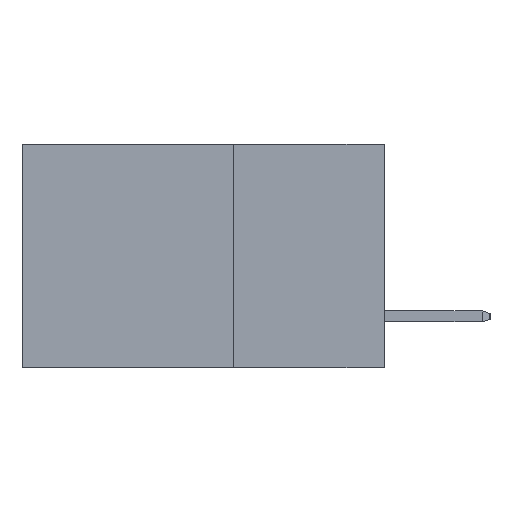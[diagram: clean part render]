
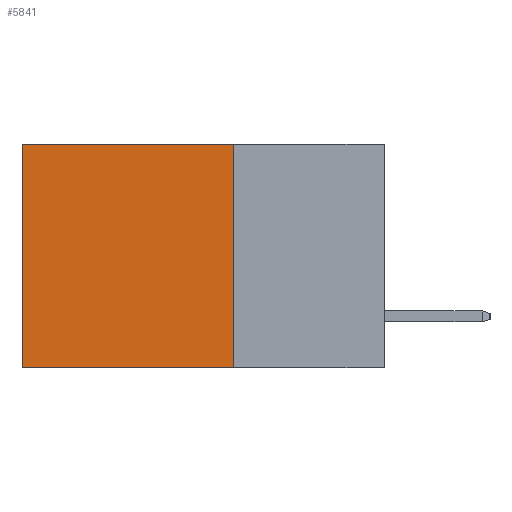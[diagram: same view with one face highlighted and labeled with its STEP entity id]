
A CAD part, left-side view. The second image highlights one B-rep face of the part: STEP entity #5841.
In plain terms, the highlighted planar face has unit normal (-1, 0, 0).
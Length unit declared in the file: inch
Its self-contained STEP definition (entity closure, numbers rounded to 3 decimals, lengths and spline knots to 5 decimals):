
#678 = CARTESIAN_POINT ( 'NONE',  ( 0.2615, 0.6, 0. ) ) ;
#769 = ORIENTED_EDGE ( 'NONE', *, *, #10296, .T. ) ;
#1385 = DIRECTION ( 'NONE',  ( 0., 0., -1. ) ) ;
#1438 = DIRECTION ( 'NONE',  ( 1., 0., 0. ) ) ;
#1522 = PLANE ( 'NONE',  #4509 ) ;
#1677 = ORIENTED_EDGE ( 'NONE', *, *, #14026, .F. ) ;
#2131 = VECTOR ( 'NONE', #11616, 39.37008 ) ;
#2308 = CARTESIAN_POINT ( 'NONE',  ( 0.2615, 0.25, -0.37 ) ) ;
#2536 = EDGE_CURVE ( 'NONE', #17397, #6190, #6015, .T. ) ;
#4198 = EDGE_CURVE ( 'NONE', #18920, #18972, #10776, .T. ) ;
#4496 = LINE ( 'NONE', #11755, #15851 ) ;
#4509 = AXIS2_PLACEMENT_3D ( 'NONE', #2308, #1438, #1385 ) ;
#5029 = CARTESIAN_POINT ( 'NONE',  ( 0.2615, 0.25, 0. ) ) ;
#5841 = ADVANCED_FACE ( 'NONE', ( #13977 ), #1522, .F. ) ;
#6015 = LINE ( 'NONE', #11828, #2131 ) ;
#6190 = VERTEX_POINT ( 'NONE', #11806 ) ;
#6911 = DIRECTION ( 'NONE',  ( 0., 0., -1. ) ) ;
#6940 = ORIENTED_EDGE ( 'NONE', *, *, #4198, .T. ) ;
#7464 = CARTESIAN_POINT ( 'NONE',  ( 0.2615, 0.25, 0. ) ) ;
#8013 = CARTESIAN_POINT ( 'NONE',  ( 0.2615, 0.6, -0.37 ) ) ;
#8168 = DIRECTION ( 'NONE',  ( 0., 1., 0. ) ) ;
#10296 = EDGE_CURVE ( 'NONE', #18972, #6190, #17639, .T. ) ;
#10776 = LINE ( 'NONE', #7464, #17719 ) ;
#11616 = DIRECTION ( 'NONE',  ( 0., 1., 0. ) ) ;
#11755 = CARTESIAN_POINT ( 'NONE',  ( 0.2615, 0.25, -0.37 ) ) ;
#11806 = CARTESIAN_POINT ( 'NONE',  ( 0.2615, 0.6, -0.37 ) ) ;
#11828 = CARTESIAN_POINT ( 'NONE',  ( 0.2615, 0.25, -0.37 ) ) ;
#12674 = CARTESIAN_POINT ( 'NONE',  ( 0.2615, 0.25, -0.37 ) ) ;
#13218 = EDGE_LOOP ( 'NONE', ( #769, #14339, #1677, #6940 ) ) ;
#13240 = DIRECTION ( 'NONE',  ( 0., 0., -1. ) ) ;
#13977 = FACE_OUTER_BOUND ( 'NONE', #13218, .T. ) ;
#14026 = EDGE_CURVE ( 'NONE', #18920, #17397, #4496, .T. ) ;
#14339 = ORIENTED_EDGE ( 'NONE', *, *, #2536, .F. ) ;
#15598 = VECTOR ( 'NONE', #6911, 39.37008 ) ;
#15851 = VECTOR ( 'NONE', #13240, 39.37008 ) ;
#17397 = VERTEX_POINT ( 'NONE', #12674 ) ;
#17639 = LINE ( 'NONE', #8013, #15598 ) ;
#17719 = VECTOR ( 'NONE', #8168, 39.37008 ) ;
#18920 = VERTEX_POINT ( 'NONE', #5029 ) ;
#18972 = VERTEX_POINT ( 'NONE', #678 ) ;
